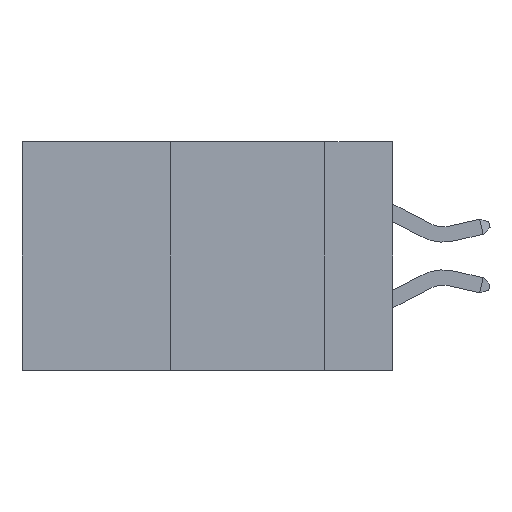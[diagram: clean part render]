
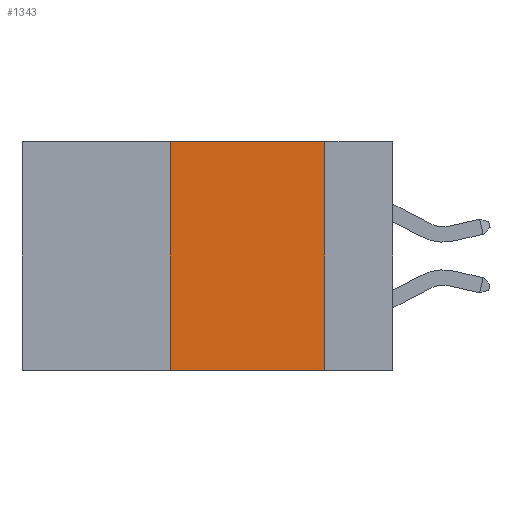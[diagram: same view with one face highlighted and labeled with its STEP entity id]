
A CAD part, left-side view. The second image highlights one B-rep face of the part: STEP entity #1343.
In plain terms, the highlighted planar face has unit normal (-1, 0, 0).
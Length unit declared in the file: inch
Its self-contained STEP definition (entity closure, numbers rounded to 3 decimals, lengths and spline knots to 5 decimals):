
#1145 = DIRECTION ( 'NONE',  ( 0., 0., 1. ) ) ;
#1343 = ADVANCED_FACE ( 'NONE', ( #7126 ), #7960, .F. ) ;
#1666 = EDGE_CURVE ( 'NONE', #8298, #6613, #24615, .T. ) ;
#2333 = CARTESIAN_POINT ( 'NONE',  ( 0., 0.11, -0.37 ) ) ;
#3199 = ORIENTED_EDGE ( 'NONE', *, *, #16054, .F. ) ;
#3842 = DIRECTION ( 'NONE',  ( 0., -1., 0. ) ) ;
#4030 = DIRECTION ( 'NONE',  ( 1., 0., 0. ) ) ;
#4229 = VECTOR ( 'NONE', #3842, 39.37008 ) ;
#5039 = CARTESIAN_POINT ( 'NONE',  ( 0., 0.6, -0.37 ) ) ;
#6254 = CARTESIAN_POINT ( 'NONE',  ( 0., 0.11, 0. ) ) ;
#6613 = VERTEX_POINT ( 'NONE', #2333 ) ;
#7009 = ORIENTED_EDGE ( 'NONE', *, *, #11427, .F. ) ;
#7014 = DIRECTION ( 'NONE',  ( 0., -1., 0. ) ) ;
#7126 = FACE_OUTER_BOUND ( 'NONE', #15836, .T. ) ;
#7447 = CARTESIAN_POINT ( 'NONE',  ( 0., 0.36, 0. ) ) ;
#7960 = PLANE ( 'NONE',  #14434 ) ;
#8178 = CARTESIAN_POINT ( 'NONE',  ( 0., 0.36, -0.37 ) ) ;
#8298 = VERTEX_POINT ( 'NONE', #8178 ) ;
#9762 = LINE ( 'NONE', #10036, #4229 ) ;
#10036 = CARTESIAN_POINT ( 'NONE',  ( 0., 0.6, 0. ) ) ;
#10529 = EDGE_CURVE ( 'NONE', #26823, #6613, #14911, .T. ) ;
#11427 = EDGE_CURVE ( 'NONE', #24248, #26823, #9762, .T. ) ;
#12044 = CARTESIAN_POINT ( 'NONE',  ( 0., 0.36, 0. ) ) ;
#13363 = ORIENTED_EDGE ( 'NONE', *, *, #1666, .T. ) ;
#13784 = ORIENTED_EDGE ( 'NONE', *, *, #10529, .F. ) ;
#14434 = AXIS2_PLACEMENT_3D ( 'NONE', #18688, #4030, #20703 ) ;
#14911 = LINE ( 'NONE', #22014, #21095 ) ;
#15836 = EDGE_LOOP ( 'NONE', ( #13784, #7009, #3199, #13363 ) ) ;
#16054 = EDGE_CURVE ( 'NONE', #8298, #24248, #25609, .T. ) ;
#17625 = DIRECTION ( 'NONE',  ( 0., 0., -1. ) ) ;
#18688 = CARTESIAN_POINT ( 'NONE',  ( 0., 0.6, 0. ) ) ;
#20136 = VECTOR ( 'NONE', #1145, 39.37008 ) ;
#20703 = DIRECTION ( 'NONE',  ( 0., 0., -1. ) ) ;
#21095 = VECTOR ( 'NONE', #17625, 39.37008 ) ;
#22014 = CARTESIAN_POINT ( 'NONE',  ( 0., 0.11, 0. ) ) ;
#22024 = VECTOR ( 'NONE', #7014, 39.37008 ) ;
#24248 = VERTEX_POINT ( 'NONE', #12044 ) ;
#24615 = LINE ( 'NONE', #5039, #22024 ) ;
#25609 = LINE ( 'NONE', #7447, #20136 ) ;
#26823 = VERTEX_POINT ( 'NONE', #6254 ) ;
